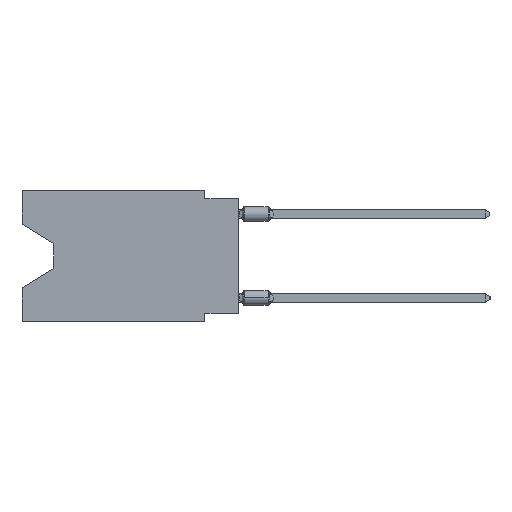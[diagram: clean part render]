
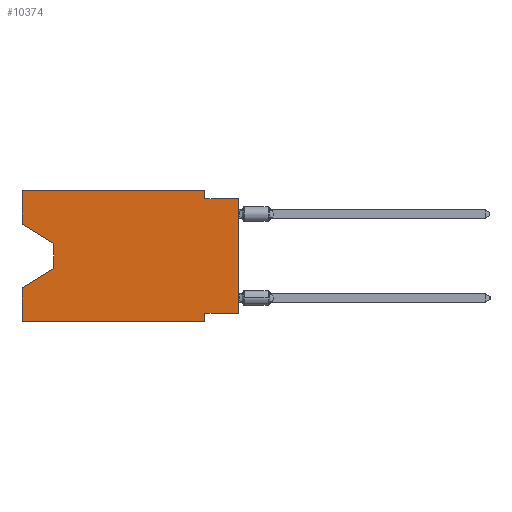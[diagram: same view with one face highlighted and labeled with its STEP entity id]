
A CAD part, left-side view. The second image highlights one B-rep face of the part: STEP entity #10374.
In plain terms, the highlighted planar face has unit normal (-1, 0, 0).
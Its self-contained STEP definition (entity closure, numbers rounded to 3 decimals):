
#465 = CARTESIAN_POINT ( 'NONE',  ( 0., 16.383, 0. ) ) ;
#1815 = CARTESIAN_POINT ( 'NONE',  ( 0., 2.54, -0.635 ) ) ;
#1838 = VERTEX_POINT ( 'NONE', #465 ) ;
#2044 = ORIENTED_EDGE ( 'NONE', *, *, #22122, .F. ) ;
#2426 = ORIENTED_EDGE ( 'NONE', *, *, #50382, .F. ) ;
#2618 = ORIENTED_EDGE ( 'NONE', *, *, #34712, .T. ) ;
#3156 = LINE ( 'NONE', #19566, #9017 ) ;
#3331 = CARTESIAN_POINT ( 'NONE',  ( 0., 2.54, 0. ) ) ;
#3935 = VECTOR ( 'NONE', #30615, 1000. ) ;
#5369 = CARTESIAN_POINT ( 'NONE',  ( 0., 13.97, -4.013 ) ) ;
#6488 = VERTEX_POINT ( 'NONE', #15596 ) ;
#6939 = DIRECTION ( 'NONE',  ( 0., 0., -1. ) ) ;
#7137 = ORIENTED_EDGE ( 'NONE', *, *, #22884, .T. ) ;
#7787 = LINE ( 'NONE', #3331, #52447 ) ;
#8406 = ORIENTED_EDGE ( 'NONE', *, *, #23574, .F. ) ;
#8742 = VECTOR ( 'NONE', #26271, 1000. ) ;
#9017 = VECTOR ( 'NONE', #54378, 1000. ) ;
#9348 = PLANE ( 'NONE',  #50789 ) ;
#9699 = EDGE_CURVE ( 'NONE', #11026, #26275, #7787, .T. ) ;
#10029 = VERTEX_POINT ( 'NONE', #20228 ) ;
#10162 = DIRECTION ( 'NONE',  ( 0., 0., -1. ) ) ;
#10374 = ADVANCED_FACE ( 'NONE', ( #18507 ), #9348, .F. ) ;
#10557 = DIRECTION ( 'NONE',  ( 0., 0., 1. ) ) ;
#11026 = VERTEX_POINT ( 'NONE', #33170 ) ;
#11650 = LINE ( 'NONE', #36963, #12329 ) ;
#12220 = CARTESIAN_POINT ( 'NONE',  ( 0., 13.97, -5.893 ) ) ;
#12329 = VECTOR ( 'NONE', #15824, 1000. ) ;
#12603 = EDGE_CURVE ( 'NONE', #40315, #6488, #15885, .T. ) ;
#12838 = LINE ( 'NONE', #22261, #29624 ) ;
#13106 = CARTESIAN_POINT ( 'NONE',  ( 0., 16.383, 0. ) ) ;
#13658 = LINE ( 'NONE', #13106, #3935 ) ;
#14167 = VERTEX_POINT ( 'NONE', #47211 ) ;
#14615 = ORIENTED_EDGE ( 'NONE', *, *, #28373, .T. ) ;
#15371 = VECTOR ( 'NONE', #36456, 1000. ) ;
#15596 = CARTESIAN_POINT ( 'NONE',  ( 0., 0., -0.635 ) ) ;
#15824 = DIRECTION ( 'NONE',  ( 0., -1., 0. ) ) ;
#15885 = LINE ( 'NONE', #53184, #15371 ) ;
#16611 = CARTESIAN_POINT ( 'NONE',  ( 0., 2.54, -9.271 ) ) ;
#17238 = CARTESIAN_POINT ( 'NONE',  ( 0., 13.97, -5.893 ) ) ;
#18507 = FACE_OUTER_BOUND ( 'NONE', #19293, .T. ) ;
#19293 = EDGE_LOOP ( 'NONE', ( #7137, #2618, #48731, #44412, #14615, #2044, #42024, #42092, #37453, #53168, #2426, #8406 ) ) ;
#19566 = CARTESIAN_POINT ( 'NONE',  ( 0., 0., -0.635 ) ) ;
#19727 = DIRECTION ( 'NONE',  ( 0., 0.855, -0.519 ) ) ;
#20061 = EDGE_CURVE ( 'NONE', #26275, #6488, #3156, .T. ) ;
#20228 = CARTESIAN_POINT ( 'NONE',  ( 0., 16.383, -9.906 ) ) ;
#20965 = CARTESIAN_POINT ( 'NONE',  ( 0., 16.383, -2.546 ) ) ;
#21061 = VECTOR ( 'NONE', #19727, 1000. ) ;
#21668 = VECTOR ( 'NONE', #49061, 1000. ) ;
#22122 = EDGE_CURVE ( 'NONE', #24258, #36742, #12838, .T. ) ;
#22261 = CARTESIAN_POINT ( 'NONE',  ( 0., 2.54, -9.906 ) ) ;
#22884 = EDGE_CURVE ( 'NONE', #39069, #14167, #28567, .T. ) ;
#23513 = EDGE_CURVE ( 'NONE', #10029, #31730, #13658, .T. ) ;
#23574 = EDGE_CURVE ( 'NONE', #39069, #1838, #36148, .T. ) ;
#24258 = VERTEX_POINT ( 'NONE', #16611 ) ;
#25190 = LINE ( 'NONE', #51089, #8742 ) ;
#25221 = CARTESIAN_POINT ( 'NONE',  ( 0., 0., -9.271 ) ) ;
#25542 = VERTEX_POINT ( 'NONE', #17238 ) ;
#26271 = DIRECTION ( 'NONE',  ( 0., -1., 0. ) ) ;
#26275 = VERTEX_POINT ( 'NONE', #1815 ) ;
#26626 = CARTESIAN_POINT ( 'NONE',  ( 0., 16.383, -7.36 ) ) ;
#28373 = EDGE_CURVE ( 'NONE', #10029, #36742, #11650, .T. ) ;
#28567 = LINE ( 'NONE', #33294, #31440 ) ;
#29624 = VECTOR ( 'NONE', #46781, 1000. ) ;
#30004 = CARTESIAN_POINT ( 'NONE',  ( 0., 2.54, -9.906 ) ) ;
#30615 = DIRECTION ( 'NONE',  ( 0., 0., 1. ) ) ;
#31298 = CARTESIAN_POINT ( 'NONE',  ( 0., 16.383, 0. ) ) ;
#31440 = VECTOR ( 'NONE', #45559, 1000. ) ;
#31730 = VERTEX_POINT ( 'NONE', #26626 ) ;
#32516 = DIRECTION ( 'NONE',  ( 0., 1., 0. ) ) ;
#33170 = CARTESIAN_POINT ( 'NONE',  ( 0., 2.54, 0. ) ) ;
#33294 = CARTESIAN_POINT ( 'NONE',  ( 0., 16.383, -2.546 ) ) ;
#34712 = EDGE_CURVE ( 'NONE', #14167, #25542, #52694, .T. ) ;
#36148 = LINE ( 'NONE', #48698, #45698 ) ;
#36456 = DIRECTION ( 'NONE',  ( 0., 0., 1. ) ) ;
#36742 = VERTEX_POINT ( 'NONE', #30004 ) ;
#36963 = CARTESIAN_POINT ( 'NONE',  ( 0., 16.383, -9.906 ) ) ;
#37453 = ORIENTED_EDGE ( 'NONE', *, *, #20061, .F. ) ;
#38619 = EDGE_CURVE ( 'NONE', #25542, #31730, #42260, .T. ) ;
#39069 = VERTEX_POINT ( 'NONE', #20965 ) ;
#40315 = VERTEX_POINT ( 'NONE', #25221 ) ;
#42024 = ORIENTED_EDGE ( 'NONE', *, *, #42681, .F. ) ;
#42092 = ORIENTED_EDGE ( 'NONE', *, *, #12603, .T. ) ;
#42260 = LINE ( 'NONE', #12220, #21061 ) ;
#42681 = EDGE_CURVE ( 'NONE', #40315, #24258, #45616, .T. ) ;
#43288 = DIRECTION ( 'NONE',  ( 1., 0., 0. ) ) ;
#44412 = ORIENTED_EDGE ( 'NONE', *, *, #23513, .F. ) ;
#45045 = CARTESIAN_POINT ( 'NONE',  ( 0., 0., -9.271 ) ) ;
#45559 = DIRECTION ( 'NONE',  ( 0., -0.855, -0.519 ) ) ;
#45616 = LINE ( 'NONE', #45045, #47418 ) ;
#45698 = VECTOR ( 'NONE', #10557, 1000. ) ;
#46781 = DIRECTION ( 'NONE',  ( 0., 0., -1. ) ) ;
#47211 = CARTESIAN_POINT ( 'NONE',  ( 0., 13.97, -4.013 ) ) ;
#47418 = VECTOR ( 'NONE', #32516, 1000. ) ;
#48698 = CARTESIAN_POINT ( 'NONE',  ( 0., 16.383, 0. ) ) ;
#48731 = ORIENTED_EDGE ( 'NONE', *, *, #38619, .T. ) ;
#49061 = DIRECTION ( 'NONE',  ( 0., 0., -1. ) ) ;
#50382 = EDGE_CURVE ( 'NONE', #1838, #11026, #25190, .T. ) ;
#50789 = AXIS2_PLACEMENT_3D ( 'NONE', #31298, #43288, #10162 ) ;
#51089 = CARTESIAN_POINT ( 'NONE',  ( 0., 16.383, 0. ) ) ;
#52447 = VECTOR ( 'NONE', #6939, 1000. ) ;
#52694 = LINE ( 'NONE', #5369, #21668 ) ;
#53168 = ORIENTED_EDGE ( 'NONE', *, *, #9699, .F. ) ;
#53184 = CARTESIAN_POINT ( 'NONE',  ( 0., 0., 0. ) ) ;
#54378 = DIRECTION ( 'NONE',  ( 0., -1., 0. ) ) ;
